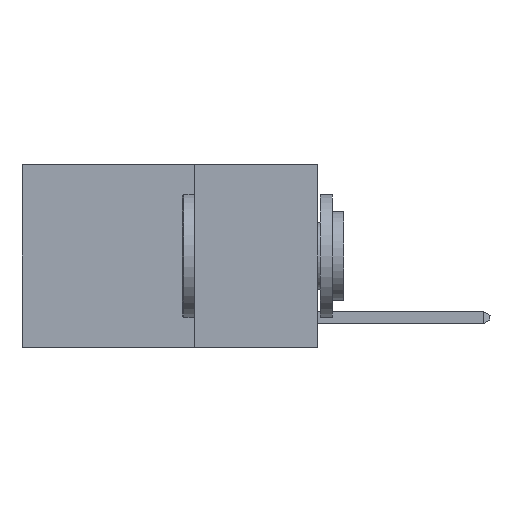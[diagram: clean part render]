
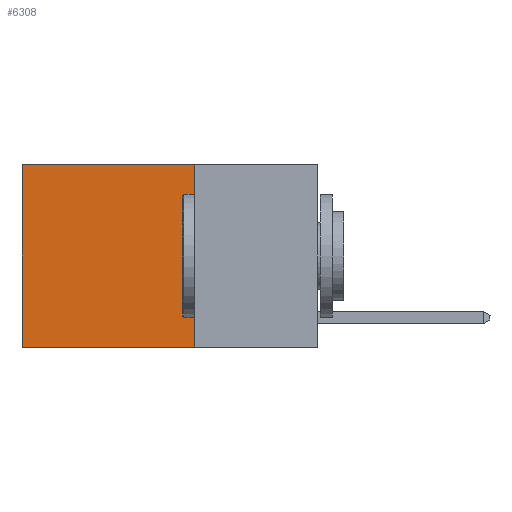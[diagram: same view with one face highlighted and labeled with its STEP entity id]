
A CAD part, left-side view. The second image highlights one B-rep face of the part: STEP entity #6308.
In plain terms, the highlighted planar face has unit normal (-1, 0, 0).
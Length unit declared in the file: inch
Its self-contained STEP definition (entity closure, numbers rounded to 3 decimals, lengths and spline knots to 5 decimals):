
#286 = VERTEX_POINT ( 'NONE', #28148 ) ;
#1299 = VERTEX_POINT ( 'NONE', #16727 ) ;
#6308 = ADVANCED_FACE ( 'NONE', ( #25361 ), #16293, .F. ) ;
#6472 = ORIENTED_EDGE ( 'NONE', *, *, #13425, .F. ) ;
#6539 = CARTESIAN_POINT ( 'NONE',  ( 0.2625, 0.25, 0. ) ) ;
#9395 = ORIENTED_EDGE ( 'NONE', *, *, #18855, .F. ) ;
#10029 = AXIS2_PLACEMENT_3D ( 'NONE', #11820, #25459, #11923 ) ;
#10633 = DIRECTION ( 'NONE',  ( 0., 1., 0. ) ) ;
#11642 = CARTESIAN_POINT ( 'NONE',  ( 0.2625, 0.6, 0. ) ) ;
#11744 = DIRECTION ( 'NONE',  ( 0., 0., -1. ) ) ;
#11820 = CARTESIAN_POINT ( 'NONE',  ( 0.2625, 0.25, 0. ) ) ;
#11923 = DIRECTION ( 'NONE',  ( 0., 0., -1. ) ) ;
#12533 = EDGE_CURVE ( 'NONE', #28598, #286, #18823, .T. ) ;
#12878 = LINE ( 'NONE', #11642, #19771 ) ;
#13425 = EDGE_CURVE ( 'NONE', #28598, #1299, #19472, .T. ) ;
#13991 = VECTOR ( 'NONE', #18439, 39.37008 ) ;
#16293 = PLANE ( 'NONE',  #10029 ) ;
#16380 = LINE ( 'NONE', #23535, #17127 ) ;
#16480 = CARTESIAN_POINT ( 'NONE',  ( 0.2625, 0.6, -0.37 ) ) ;
#16727 = CARTESIAN_POINT ( 'NONE',  ( 0.2625, 0.25, -0.37 ) ) ;
#16732 = EDGE_LOOP ( 'NONE', ( #24869, #9395, #6472, #28831 ) ) ;
#17127 = VECTOR ( 'NONE', #25971, 39.37008 ) ;
#18439 = DIRECTION ( 'NONE',  ( 0., 0., -1. ) ) ;
#18823 = LINE ( 'NONE', #23011, #23164 ) ;
#18855 = EDGE_CURVE ( 'NONE', #1299, #25780, #16380, .T. ) ;
#19472 = LINE ( 'NONE', #20799, #13991 ) ;
#19771 = VECTOR ( 'NONE', #11744, 39.37008 ) ;
#20799 = CARTESIAN_POINT ( 'NONE',  ( 0.2625, 0.25, 0. ) ) ;
#23011 = CARTESIAN_POINT ( 'NONE',  ( 0.2625, 0.25, 0. ) ) ;
#23164 = VECTOR ( 'NONE', #10633, 39.37008 ) ;
#23535 = CARTESIAN_POINT ( 'NONE',  ( 0.2625, 0.25, -0.37 ) ) ;
#24869 = ORIENTED_EDGE ( 'NONE', *, *, #25469, .T. ) ;
#25361 = FACE_OUTER_BOUND ( 'NONE', #16732, .T. ) ;
#25459 = DIRECTION ( 'NONE',  ( 1., 0., 0. ) ) ;
#25469 = EDGE_CURVE ( 'NONE', #286, #25780, #12878, .T. ) ;
#25780 = VERTEX_POINT ( 'NONE', #16480 ) ;
#25971 = DIRECTION ( 'NONE',  ( 0., 1., 0. ) ) ;
#28148 = CARTESIAN_POINT ( 'NONE',  ( 0.2625, 0.6, 0. ) ) ;
#28598 = VERTEX_POINT ( 'NONE', #6539 ) ;
#28831 = ORIENTED_EDGE ( 'NONE', *, *, #12533, .T. ) ;
